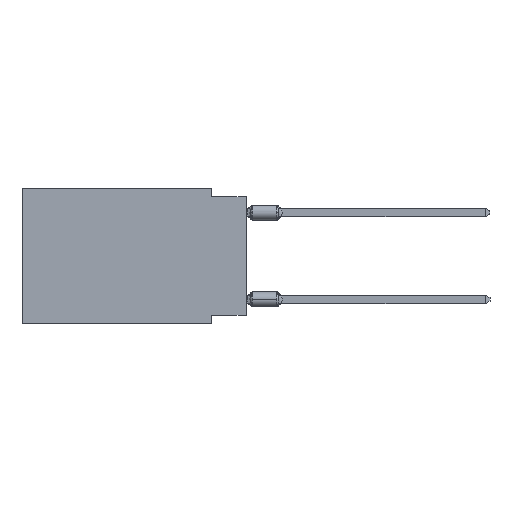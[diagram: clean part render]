
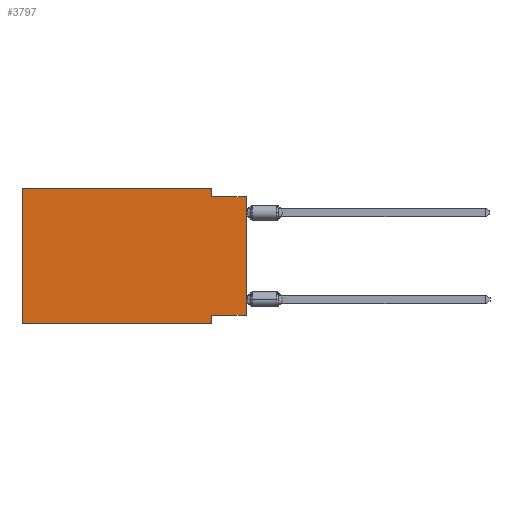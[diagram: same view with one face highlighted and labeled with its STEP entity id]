
A CAD part, left-side view. The second image highlights one B-rep face of the part: STEP entity #3797.
In plain terms, the highlighted planar face has unit normal (-1, 0, 0).
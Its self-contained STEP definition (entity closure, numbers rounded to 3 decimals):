
#37 = LINE ( 'NONE', #5473, #21955 ) ;
#371 = VECTOR ( 'NONE', #22274, 1000. ) ;
#519 = VERTEX_POINT ( 'NONE', #2307 ) ;
#758 = LINE ( 'NONE', #14038, #9797 ) ;
#2165 = VERTEX_POINT ( 'NONE', #12420 ) ;
#2307 = CARTESIAN_POINT ( 'NONE',  ( 0., 2.54, -0.635 ) ) ;
#2367 = EDGE_CURVE ( 'NONE', #2165, #4454, #13970, .T. ) ;
#3388 = AXIS2_PLACEMENT_3D ( 'NONE', #12510, #5158, #12393 ) ;
#3797 = ADVANCED_FACE ( 'NONE', ( #14009 ), #20907, .F. ) ;
#4454 = VERTEX_POINT ( 'NONE', #15643 ) ;
#4623 = DIRECTION ( 'NONE',  ( 0., 0., 1. ) ) ;
#4796 = CARTESIAN_POINT ( 'NONE',  ( 0., 2.54, -9.271 ) ) ;
#5158 = DIRECTION ( 'NONE',  ( 1., 0., 0. ) ) ;
#5241 = DIRECTION ( 'NONE',  ( 0., -1., 0. ) ) ;
#5323 = ORIENTED_EDGE ( 'NONE', *, *, #17188, .T. ) ;
#5473 = CARTESIAN_POINT ( 'NONE',  ( 0., 16.383, -9.906 ) ) ;
#5701 = VECTOR ( 'NONE', #13197, 1000. ) ;
#6186 = ORIENTED_EDGE ( 'NONE', *, *, #21732, .F. ) ;
#6237 = LINE ( 'NONE', #20366, #13530 ) ;
#6439 = CARTESIAN_POINT ( 'NONE',  ( 0., 16.383, -9.906 ) ) ;
#6539 = ORIENTED_EDGE ( 'NONE', *, *, #12213, .T. ) ;
#6754 = ORIENTED_EDGE ( 'NONE', *, *, #19766, .F. ) ;
#6853 = VECTOR ( 'NONE', #21227, 1000. ) ;
#7162 = VERTEX_POINT ( 'NONE', #6439 ) ;
#8028 = EDGE_LOOP ( 'NONE', ( #6539, #8282, #6186, #11192, #22066, #5323, #6754, #10180 ) ) ;
#8282 = ORIENTED_EDGE ( 'NONE', *, *, #21194, .F. ) ;
#9797 = VECTOR ( 'NONE', #14684, 1000. ) ;
#9825 = CARTESIAN_POINT ( 'NONE',  ( 0., 0., -0.635 ) ) ;
#10013 = CARTESIAN_POINT ( 'NONE',  ( 0., 2.54, 0. ) ) ;
#10180 = ORIENTED_EDGE ( 'NONE', *, *, #22705, .F. ) ;
#11192 = ORIENTED_EDGE ( 'NONE', *, *, #2367, .F. ) ;
#12213 = EDGE_CURVE ( 'NONE', #18187, #12377, #758, .T. ) ;
#12377 = VERTEX_POINT ( 'NONE', #9825 ) ;
#12393 = DIRECTION ( 'NONE',  ( 0., 0., -1. ) ) ;
#12420 = CARTESIAN_POINT ( 'NONE',  ( 0., 16.383, 0. ) ) ;
#12510 = CARTESIAN_POINT ( 'NONE',  ( 0., 16.383, 0. ) ) ;
#12605 = LINE ( 'NONE', #12714, #6853 ) ;
#12714 = CARTESIAN_POINT ( 'NONE',  ( 0., 0., -9.271 ) ) ;
#13197 = DIRECTION ( 'NONE',  ( 0., -1., 0. ) ) ;
#13530 = VECTOR ( 'NONE', #4623, 1000. ) ;
#13970 = LINE ( 'NONE', #17073, #371 ) ;
#14009 = FACE_OUTER_BOUND ( 'NONE', #8028, .T. ) ;
#14038 = CARTESIAN_POINT ( 'NONE',  ( 0., 0., 0. ) ) ;
#14304 = VERTEX_POINT ( 'NONE', #4796 ) ;
#14598 = CARTESIAN_POINT ( 'NONE',  ( 0., 2.54, -9.906 ) ) ;
#14684 = DIRECTION ( 'NONE',  ( 0., 0., 1. ) ) ;
#15643 = CARTESIAN_POINT ( 'NONE',  ( 0., 2.54, 0. ) ) ;
#15725 = LINE ( 'NONE', #17107, #17069 ) ;
#17069 = VECTOR ( 'NONE', #21122, 1000. ) ;
#17073 = CARTESIAN_POINT ( 'NONE',  ( 0., 16.383, 0. ) ) ;
#17107 = CARTESIAN_POINT ( 'NONE',  ( 0., 2.54, -9.906 ) ) ;
#17188 = EDGE_CURVE ( 'NONE', #7162, #20627, #37, .T. ) ;
#18187 = VERTEX_POINT ( 'NONE', #21780 ) ;
#18420 = EDGE_CURVE ( 'NONE', #7162, #2165, #6237, .T. ) ;
#19766 = EDGE_CURVE ( 'NONE', #14304, #20627, #15725, .T. ) ;
#20200 = CARTESIAN_POINT ( 'NONE',  ( 0., 0., -0.635 ) ) ;
#20366 = CARTESIAN_POINT ( 'NONE',  ( 0., 16.383, 0. ) ) ;
#20627 = VERTEX_POINT ( 'NONE', #14598 ) ;
#20845 = LINE ( 'NONE', #10013, #21880 ) ;
#20907 = PLANE ( 'NONE',  #3388 ) ;
#21122 = DIRECTION ( 'NONE',  ( 0., 0., -1. ) ) ;
#21194 = EDGE_CURVE ( 'NONE', #519, #12377, #22055, .T. ) ;
#21227 = DIRECTION ( 'NONE',  ( 0., 1., 0. ) ) ;
#21732 = EDGE_CURVE ( 'NONE', #4454, #519, #20845, .T. ) ;
#21780 = CARTESIAN_POINT ( 'NONE',  ( 0., 0., -9.271 ) ) ;
#21880 = VECTOR ( 'NONE', #22365, 1000. ) ;
#21955 = VECTOR ( 'NONE', #5241, 1000. ) ;
#22055 = LINE ( 'NONE', #20200, #5701 ) ;
#22066 = ORIENTED_EDGE ( 'NONE', *, *, #18420, .F. ) ;
#22274 = DIRECTION ( 'NONE',  ( 0., -1., 0. ) ) ;
#22365 = DIRECTION ( 'NONE',  ( 0., 0., -1. ) ) ;
#22705 = EDGE_CURVE ( 'NONE', #18187, #14304, #12605, .T. ) ;
